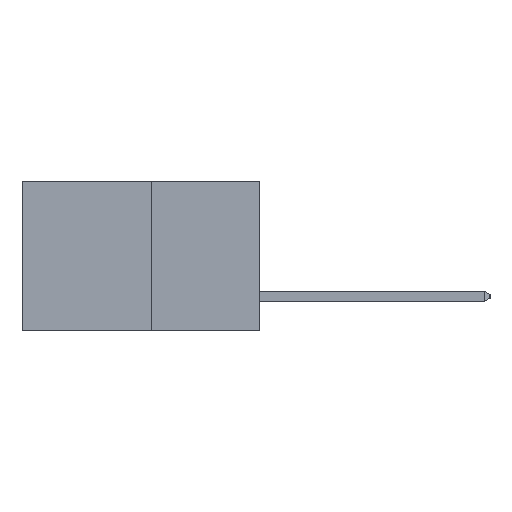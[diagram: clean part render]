
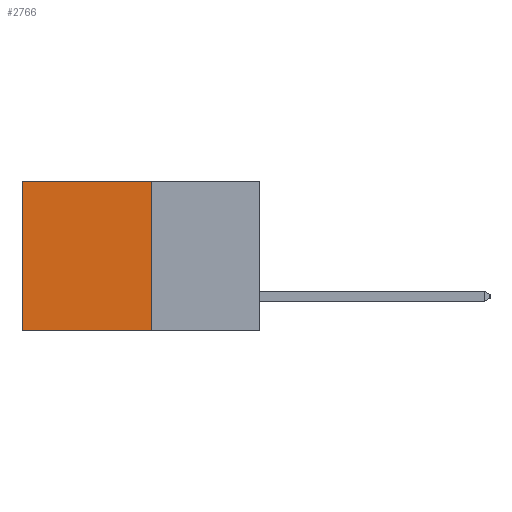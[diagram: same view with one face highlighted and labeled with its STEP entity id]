
A CAD part, left-side view. The second image highlights one B-rep face of the part: STEP entity #2766.
In plain terms, the highlighted planar face has unit normal (-1, 0, 0).
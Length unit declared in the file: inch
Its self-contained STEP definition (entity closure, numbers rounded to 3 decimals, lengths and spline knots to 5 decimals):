
#12 = EDGE_CURVE ( 'NONE', #1623, #18898, #6627, .T. ) ;
#56 = CARTESIAN_POINT ( 'NONE',  ( 0.277, 0.27, -0.37 ) ) ;
#473 = DIRECTION ( 'NONE',  ( 0., 0., -1. ) ) ;
#1340 = VECTOR ( 'NONE', #13578, 39.37008 ) ;
#1623 = VERTEX_POINT ( 'NONE', #7280 ) ;
#2545 = LINE ( 'NONE', #12327, #7170 ) ;
#2594 = DIRECTION ( 'NONE',  ( 0., 1., 0. ) ) ;
#2766 = ADVANCED_FACE ( 'NONE', ( #20399 ), #21834, .F. ) ;
#3873 = EDGE_CURVE ( 'NONE', #1623, #24169, #7083, .T. ) ;
#4630 = VECTOR ( 'NONE', #2594, 39.37008 ) ;
#6627 = LINE ( 'NONE', #12951, #1340 ) ;
#7083 = LINE ( 'NONE', #56, #11525 ) ;
#7170 = VECTOR ( 'NONE', #12415, 39.37008 ) ;
#7280 = CARTESIAN_POINT ( 'NONE',  ( 0.277, 0.27, 0. ) ) ;
#7329 = EDGE_CURVE ( 'NONE', #18898, #7540, #2545, .T. ) ;
#7540 = VERTEX_POINT ( 'NONE', #21925 ) ;
#7716 = ORIENTED_EDGE ( 'NONE', *, *, #12, .T. ) ;
#7870 = ORIENTED_EDGE ( 'NONE', *, *, #9849, .F. ) ;
#8275 = EDGE_LOOP ( 'NONE', ( #11449, #7870, #15648, #7716 ) ) ;
#9849 = EDGE_CURVE ( 'NONE', #24169, #7540, #19524, .T. ) ;
#11449 = ORIENTED_EDGE ( 'NONE', *, *, #7329, .T. ) ;
#11525 = VECTOR ( 'NONE', #473, 39.37008 ) ;
#12327 = CARTESIAN_POINT ( 'NONE',  ( 0.277, 0.59, -0.37 ) ) ;
#12415 = DIRECTION ( 'NONE',  ( 0., 0., -1. ) ) ;
#12951 = CARTESIAN_POINT ( 'NONE',  ( 0.277, 0.27, 0. ) ) ;
#13578 = DIRECTION ( 'NONE',  ( 0., 1., 0. ) ) ;
#14119 = CARTESIAN_POINT ( 'NONE',  ( 0.277, 0.27, -0.37 ) ) ;
#15648 = ORIENTED_EDGE ( 'NONE', *, *, #3873, .F. ) ;
#18058 = DIRECTION ( 'NONE',  ( 0., 0., -1. ) ) ;
#18898 = VERTEX_POINT ( 'NONE', #22682 ) ;
#19524 = LINE ( 'NONE', #14119, #4630 ) ;
#20399 = FACE_OUTER_BOUND ( 'NONE', #8275, .T. ) ;
#20764 = CARTESIAN_POINT ( 'NONE',  ( 0.277, 0.27, -0.37 ) ) ;
#21834 = PLANE ( 'NONE',  #22289 ) ;
#21925 = CARTESIAN_POINT ( 'NONE',  ( 0.277, 0.59, -0.37 ) ) ;
#21932 = DIRECTION ( 'NONE',  ( 1., 0., 0. ) ) ;
#22289 = AXIS2_PLACEMENT_3D ( 'NONE', #20764, #21932, #18058 ) ;
#22682 = CARTESIAN_POINT ( 'NONE',  ( 0.277, 0.59, 0. ) ) ;
#23904 = CARTESIAN_POINT ( 'NONE',  ( 0.277, 0.27, -0.37 ) ) ;
#24169 = VERTEX_POINT ( 'NONE', #23904 ) ;
